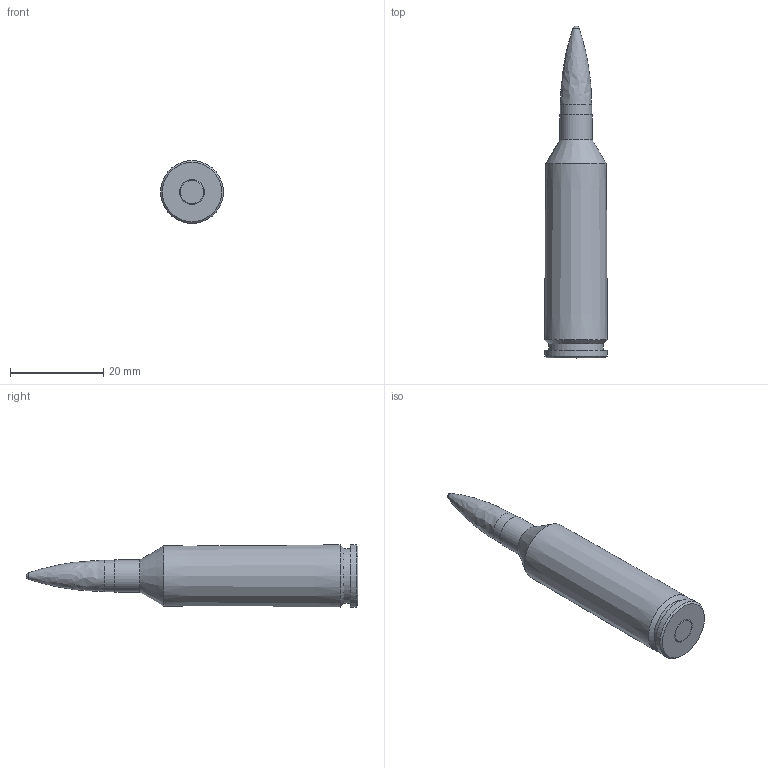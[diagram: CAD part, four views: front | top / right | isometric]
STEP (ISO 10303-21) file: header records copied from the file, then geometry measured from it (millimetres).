
FILE_DESCRIPTION((''),'2;1');
FILE_NAME('6.17 SPITFIRE.stp','2012-11-29T12:38:49',('agarrett'),(''),'Autodesk Inventor 2012','Autodesk Inventor 2012','');
FILE_SCHEMA(('AUTOMOTIVE_DESIGN { 1 0 10303 214 1 1 1 1 }'));
Length unit declared in the file: inch
Products named in the file (4): iLogic Cartridge; Rimless Bottleneck; iLogic SP Bullet; PRIMER
Assembly tree (3 placements, depth 2):
  iLogic Cartridge
    Rimless Bottleneck
    iLogic SP Bullet
    PRIMER
Bounding box: 13.46 x 71.12 x 13.46 mm (x, y, z)
Volume: 7105.3 mm3; surface area: 3070.7 mm2
Topology: 3 solids, 3 shells, 27 faces, 41 edges, 24 vertices
Faces by surface type: plane 9, cylinder 8, cone 4, torus 4, sphere 1, bspline 1
Full cylindrical faces by diameter (mm): 1.778 x1, 5.08 x1, 5.334 x2, 6.68 x1, 6.985 x1, 11.684 x1, 13.462 x1
Entity records: 670 total; most frequent: DIRECTION 114, CARTESIAN_POINT 108, AXIS2_PLACEMENT_3D 57, ORIENTED_EDGE 48, EDGE_LOOP 48, FACE_OUTER_BOUND 27, ADVANCED_FACE 27, VERTEX_POINT 24
